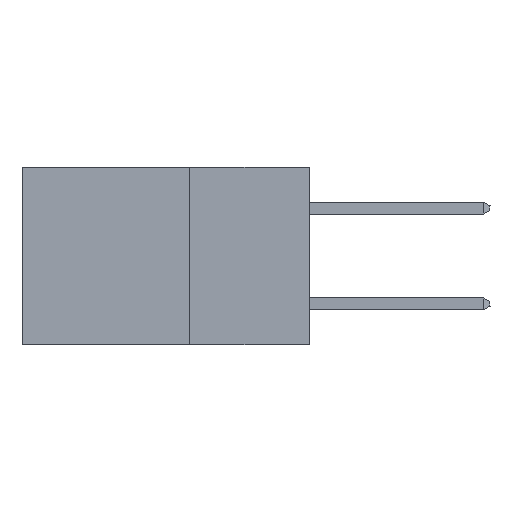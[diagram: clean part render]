
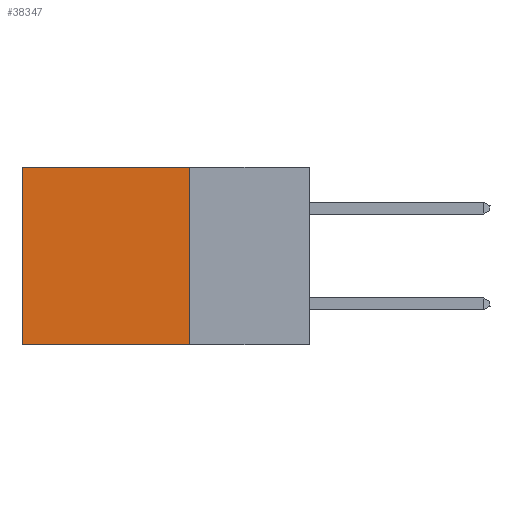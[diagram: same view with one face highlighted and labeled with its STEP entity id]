
A CAD part, left-side view. The second image highlights one B-rep face of the part: STEP entity #38347.
In plain terms, the highlighted planar face has unit normal (-1, 0, 0).
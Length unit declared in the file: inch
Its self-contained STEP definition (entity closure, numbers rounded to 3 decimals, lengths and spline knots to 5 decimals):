
#307 = CARTESIAN_POINT ( 'NONE',  ( 0.2875, 0.6, 0. ) ) ;
#2028 = VERTEX_POINT ( 'NONE', #10704 ) ;
#3134 = CARTESIAN_POINT ( 'NONE',  ( 0.2875, 0.25, -0.37 ) ) ;
#3288 = VERTEX_POINT ( 'NONE', #31967 ) ;
#6138 = CARTESIAN_POINT ( 'NONE',  ( 0.2875, 0.25, 0. ) ) ;
#7451 = DIRECTION ( 'NONE',  ( 0., 0., -1. ) ) ;
#7474 = VECTOR ( 'NONE', #42969, 39.37008 ) ;
#8161 = DIRECTION ( 'NONE',  ( 1., 0., 0. ) ) ;
#8214 = VECTOR ( 'NONE', #27975, 39.37008 ) ;
#10531 = ORIENTED_EDGE ( 'NONE', *, *, #24147, .F. ) ;
#10704 = CARTESIAN_POINT ( 'NONE',  ( 0.2875, 0.6, 0. ) ) ;
#11932 = VECTOR ( 'NONE', #27325, 39.37008 ) ;
#12521 = EDGE_CURVE ( 'NONE', #26589, #2028, #16663, .T. ) ;
#16663 = LINE ( 'NONE', #25708, #7474 ) ;
#18417 = CARTESIAN_POINT ( 'NONE',  ( 0.2875, 0.25, 0. ) ) ;
#20721 = AXIS2_PLACEMENT_3D ( 'NONE', #18417, #8161, #32281 ) ;
#22110 = EDGE_CURVE ( 'NONE', #2028, #25350, #35725, .T. ) ;
#22168 = LINE ( 'NONE', #3134, #11932 ) ;
#22687 = EDGE_CURVE ( 'NONE', #3288, #25350, #22168, .T. ) ;
#24147 = EDGE_CURVE ( 'NONE', #26589, #3288, #27999, .T. ) ;
#25350 = VERTEX_POINT ( 'NONE', #37271 ) ;
#25708 = CARTESIAN_POINT ( 'NONE',  ( 0.2875, 0.25, 0. ) ) ;
#26051 = ORIENTED_EDGE ( 'NONE', *, *, #12521, .T. ) ;
#26217 = ORIENTED_EDGE ( 'NONE', *, *, #22110, .T. ) ;
#26589 = VERTEX_POINT ( 'NONE', #6138 ) ;
#27325 = DIRECTION ( 'NONE',  ( 0., 1., 0. ) ) ;
#27975 = DIRECTION ( 'NONE',  ( 0., 0., -1. ) ) ;
#27999 = LINE ( 'NONE', #31566, #44147 ) ;
#28673 = PLANE ( 'NONE',  #20721 ) ;
#31566 = CARTESIAN_POINT ( 'NONE',  ( 0.2875, 0.25, 0. ) ) ;
#31967 = CARTESIAN_POINT ( 'NONE',  ( 0.2875, 0.25, -0.37 ) ) ;
#32281 = DIRECTION ( 'NONE',  ( 0., 0., -1. ) ) ;
#35280 = ORIENTED_EDGE ( 'NONE', *, *, #22687, .F. ) ;
#35725 = LINE ( 'NONE', #307, #8214 ) ;
#37271 = CARTESIAN_POINT ( 'NONE',  ( 0.2875, 0.6, -0.37 ) ) ;
#38347 = ADVANCED_FACE ( 'NONE', ( #41893 ), #28673, .F. ) ;
#40106 = EDGE_LOOP ( 'NONE', ( #26217, #35280, #10531, #26051 ) ) ;
#41893 = FACE_OUTER_BOUND ( 'NONE', #40106, .T. ) ;
#42969 = DIRECTION ( 'NONE',  ( 0., 1., 0. ) ) ;
#44147 = VECTOR ( 'NONE', #7451, 39.37008 ) ;
